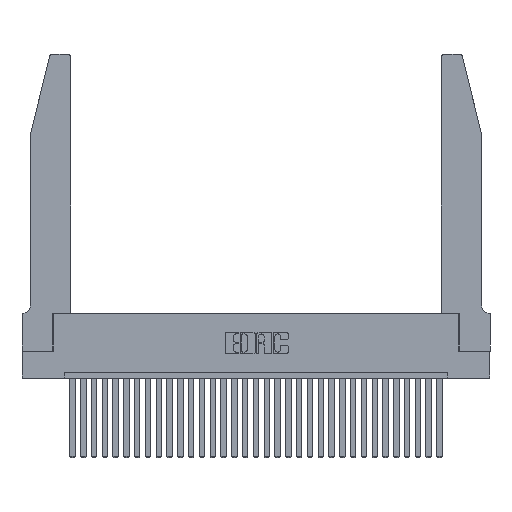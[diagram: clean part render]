
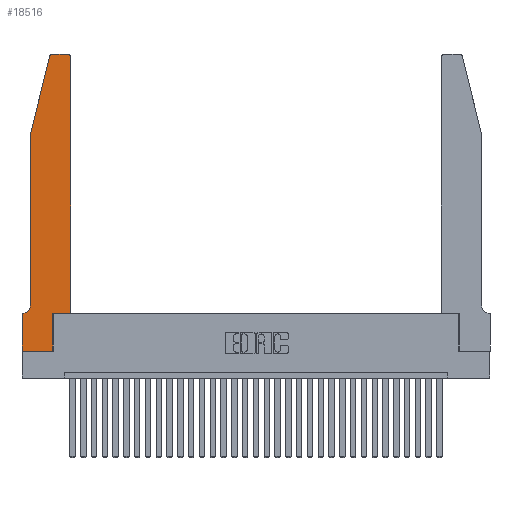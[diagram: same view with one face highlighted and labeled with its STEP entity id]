
A CAD part, top view. The second image highlights one B-rep face of the part: STEP entity #18516.
In plain terms, the highlighted planar face has unit normal (0, 0, 1).
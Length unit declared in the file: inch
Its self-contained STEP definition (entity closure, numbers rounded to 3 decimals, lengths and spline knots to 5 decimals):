
#187 = ORIENTED_EDGE ( 'NONE', *, *, #16091, .T. ) ;
#210 = LINE ( 'NONE', #24975, #2851 ) ;
#791 = CARTESIAN_POINT ( 'NONE',  ( 0., 0.35, 0.37 ) ) ;
#796 = CARTESIAN_POINT ( 'NONE',  ( 0.0755, 0.35, 0.37 ) ) ;
#902 = DIRECTION ( 'NONE',  ( 0., 0., 1. ) ) ;
#1170 = CARTESIAN_POINT ( 'NONE',  ( 0., 0.35, 0.37 ) ) ;
#2299 = ORIENTED_EDGE ( 'NONE', *, *, #24596, .T. ) ;
#2371 = EDGE_CURVE ( 'NONE', #12979, #28736, #7517, .T. ) ;
#2527 = ORIENTED_EDGE ( 'NONE', *, *, #7968, .T. ) ;
#2652 = VECTOR ( 'NONE', #31261, 39.37008 ) ;
#2851 = VECTOR ( 'NONE', #14882, 39.37008 ) ;
#2985 = CARTESIAN_POINT ( 'NONE',  ( 0.0755, 2., 0.37 ) ) ;
#3195 = VECTOR ( 'NONE', #9010, 39.37008 ) ;
#3796 = VERTEX_POINT ( 'NONE', #16923 ) ;
#3911 = ORIENTED_EDGE ( 'NONE', *, *, #31085, .T. ) ;
#4377 = DIRECTION ( 'NONE',  ( 1., 0., 0. ) ) ;
#4533 = CARTESIAN_POINT ( 'NONE',  ( 0.284, 2.72, 0.37 ) ) ;
#5021 = CARTESIAN_POINT ( 'NONE',  ( 0.0755, 2., 0.37 ) ) ;
#5751 = PLANE ( 'NONE',  #31040 ) ;
#6042 = VECTOR ( 'NONE', #10598, 39.37008 ) ;
#6396 = EDGE_CURVE ( 'NONE', #25121, #13026, #25549, .T. ) ;
#7012 = CIRCLE ( 'NONE', #10353, 0.07 ) ;
#7196 = ORIENTED_EDGE ( 'NONE', *, *, #15657, .T. ) ;
#7517 = LINE ( 'NONE', #11503, #12232 ) ;
#7820 = VERTEX_POINT ( 'NONE', #20094 ) ;
#7928 = DIRECTION ( 'NONE',  ( 0., 0., 1. ) ) ;
#7968 = EDGE_CURVE ( 'NONE', #20983, #16973, #10855, .T. ) ;
#8488 = CARTESIAN_POINT ( 'NONE',  ( 0.0755, 0.42, 0.37 ) ) ;
#8621 = ORIENTED_EDGE ( 'NONE', *, *, #26580, .T. ) ;
#8627 = FACE_OUTER_BOUND ( 'NONE', #15078, .T. ) ;
#8714 = EDGE_CURVE ( 'NONE', #16973, #31316, #16599, .T. ) ;
#9010 = DIRECTION ( 'NONE',  ( -1., 0., 0. ) ) ;
#9140 = CARTESIAN_POINT ( 'NONE',  ( 0., 0., 0.37 ) ) ;
#9402 = ORIENTED_EDGE ( 'NONE', *, *, #15939, .T. ) ;
#9444 = DIRECTION ( 'NONE',  ( -0.239, -0.971, 0. ) ) ;
#9700 = VERTEX_POINT ( 'NONE', #1170 ) ;
#9824 = ORIENTED_EDGE ( 'NONE', *, *, #2371, .T. ) ;
#10072 = CIRCLE ( 'NONE', #18267, 0.03 ) ;
#10353 = AXIS2_PLACEMENT_3D ( 'NONE', #24520, #27022, #27495 ) ;
#10574 = CARTESIAN_POINT ( 'NONE',  ( 0.4205, 2.75, 0.37 ) ) ;
#10598 = DIRECTION ( 'NONE',  ( 0., 1., 0. ) ) ;
#10734 = LINE ( 'NONE', #23795, #19611 ) ;
#10855 = LINE ( 'NONE', #19131, #2652 ) ;
#11409 = LINE ( 'NONE', #796, #3195 ) ;
#11503 = CARTESIAN_POINT ( 'NONE',  ( 0.2605, 2.75, 0.37 ) ) ;
#11605 = VECTOR ( 'NONE', #28845, 39.37008 ) ;
#11822 = LINE ( 'NONE', #29741, #19072 ) ;
#12232 = VECTOR ( 'NONE', #30924, 39.37008 ) ;
#12567 = VERTEX_POINT ( 'NONE', #16487 ) ;
#12979 = VERTEX_POINT ( 'NONE', #10574 ) ;
#13026 = VERTEX_POINT ( 'NONE', #8488 ) ;
#13203 = ORIENTED_EDGE ( 'NONE', *, *, #6396, .T. ) ;
#13782 = AXIS2_PLACEMENT_3D ( 'NONE', #4533, #21526, #21842 ) ;
#14594 = DIRECTION ( 'NONE',  ( 0., -1., 0. ) ) ;
#14882 = DIRECTION ( 'NONE',  ( 0., -1., 0. ) ) ;
#15078 = EDGE_LOOP ( 'NONE', ( #9824, #25234, #2299, #13203, #7196, #8621, #3911, #2527, #21116, #187, #26076, #9402 ) ) ;
#15657 = EDGE_CURVE ( 'NONE', #13026, #3796, #7012, .T. ) ;
#15939 = EDGE_CURVE ( 'NONE', #7820, #12979, #10072, .T. ) ;
#16091 = EDGE_CURVE ( 'NONE', #31316, #19137, #11822, .T. ) ;
#16487 = CARTESIAN_POINT ( 'NONE',  ( 0.25487, 2.72718, 0.37 ) ) ;
#16599 = LINE ( 'NONE', #26394, #11605 ) ;
#16923 = CARTESIAN_POINT ( 'NONE',  ( 0.0055, 0.35, 0.37 ) ) ;
#16973 = VERTEX_POINT ( 'NONE', #26673 ) ;
#18267 = AXIS2_PLACEMENT_3D ( 'NONE', #30396, #7928, #23154 ) ;
#18516 = ADVANCED_FACE ( 'NONE', ( #8627 ), #5751, .T. ) ;
#19072 = VECTOR ( 'NONE', #4377, 39.37008 ) ;
#19131 = CARTESIAN_POINT ( 'NONE',  ( 0., 0., 0.37 ) ) ;
#19137 = VERTEX_POINT ( 'NONE', #22629 ) ;
#19611 = VECTOR ( 'NONE', #9444, 39.37008 ) ;
#20094 = CARTESIAN_POINT ( 'NONE',  ( 0.4505, 2.72, 0.37 ) ) ;
#20983 = VERTEX_POINT ( 'NONE', #9140 ) ;
#21116 = ORIENTED_EDGE ( 'NONE', *, *, #8714, .T. ) ;
#21127 = CARTESIAN_POINT ( 'NONE',  ( 0.2865, 0.35, 0.37 ) ) ;
#21526 = DIRECTION ( 'NONE',  ( 0., 0., 1. ) ) ;
#21842 = DIRECTION ( 'NONE',  ( 1., 0., 0. ) ) ;
#22305 = EDGE_CURVE ( 'NONE', #19137, #7820, #29183, .T. ) ;
#22629 = CARTESIAN_POINT ( 'NONE',  ( 0.4505, 0.35, 0.37 ) ) ;
#23154 = DIRECTION ( 'NONE',  ( 1., 0., 0. ) ) ;
#23651 = VECTOR ( 'NONE', #14594, 39.37008 ) ;
#23795 = CARTESIAN_POINT ( 'NONE',  ( 0.0755, 2., 0.37 ) ) ;
#24520 = CARTESIAN_POINT ( 'NONE',  ( 0.0055, 0.42, 0.37 ) ) ;
#24596 = EDGE_CURVE ( 'NONE', #12567, #25121, #10734, .T. ) ;
#24975 = CARTESIAN_POINT ( 'NONE',  ( 0., 0., 0.37 ) ) ;
#25121 = VERTEX_POINT ( 'NONE', #2985 ) ;
#25234 = ORIENTED_EDGE ( 'NONE', *, *, #26710, .T. ) ;
#25549 = LINE ( 'NONE', #5021, #23651 ) ;
#25612 = DIRECTION ( 'NONE',  ( 1., 0., 0. ) ) ;
#26012 = CIRCLE ( 'NONE', #13782, 0.03 ) ;
#26076 = ORIENTED_EDGE ( 'NONE', *, *, #22305, .T. ) ;
#26117 = CARTESIAN_POINT ( 'NONE',  ( 0.284, 2.75, 0.37 ) ) ;
#26394 = CARTESIAN_POINT ( 'NONE',  ( 0.2865, 0.35, 0.37 ) ) ;
#26580 = EDGE_CURVE ( 'NONE', #3796, #9700, #11409, .T. ) ;
#26673 = CARTESIAN_POINT ( 'NONE',  ( 0.2865, 0., 0.37 ) ) ;
#26710 = EDGE_CURVE ( 'NONE', #28736, #12567, #26012, .T. ) ;
#27022 = DIRECTION ( 'NONE',  ( 0., 0., -1. ) ) ;
#27495 = DIRECTION ( 'NONE',  ( -1., 0., 0. ) ) ;
#28736 = VERTEX_POINT ( 'NONE', #26117 ) ;
#28845 = DIRECTION ( 'NONE',  ( 0., 1., 0. ) ) ;
#29183 = LINE ( 'NONE', #29832, #6042 ) ;
#29741 = CARTESIAN_POINT ( 'NONE',  ( 0.4505, 0.35, 0.37 ) ) ;
#29832 = CARTESIAN_POINT ( 'NONE',  ( 0.4505, 0.35, 0.37 ) ) ;
#30396 = CARTESIAN_POINT ( 'NONE',  ( 0.4205, 2.72, 0.37 ) ) ;
#30924 = DIRECTION ( 'NONE',  ( -1., 0., 0. ) ) ;
#31040 = AXIS2_PLACEMENT_3D ( 'NONE', #791, #902, #25612 ) ;
#31085 = EDGE_CURVE ( 'NONE', #9700, #20983, #210, .T. ) ;
#31261 = DIRECTION ( 'NONE',  ( 1., 0., 0. ) ) ;
#31316 = VERTEX_POINT ( 'NONE', #21127 ) ;
